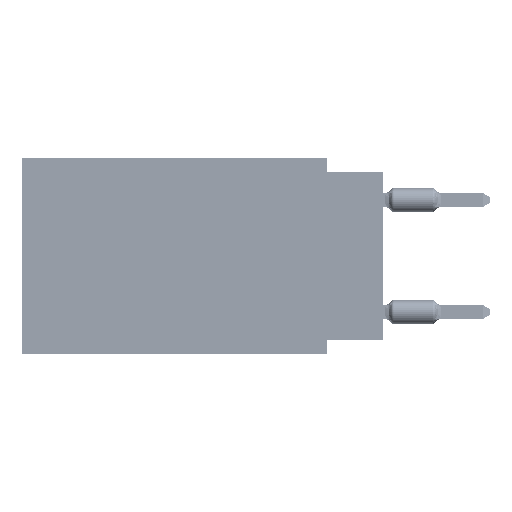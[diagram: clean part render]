
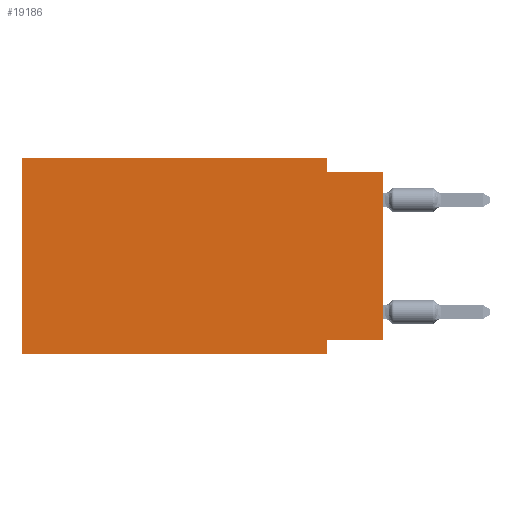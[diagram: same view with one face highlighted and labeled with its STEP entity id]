
A CAD part, left-side view. The second image highlights one B-rep face of the part: STEP entity #19186.
In plain terms, the highlighted planar face has unit normal (-1, 0, 0).
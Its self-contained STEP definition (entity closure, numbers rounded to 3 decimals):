
#31 = EDGE_CURVE ( 'NONE', #23636, #20899, #43520, .T. ) ;
#318 = DIRECTION ( 'NONE',  ( 0., -1., 0. ) ) ;
#2616 = VECTOR ( 'NONE', #43122, 1000. ) ;
#3422 = LINE ( 'NONE', #37999, #2616 ) ;
#3876 = DIRECTION ( 'NONE',  ( 0., 1., 0. ) ) ;
#4145 = VERTEX_POINT ( 'NONE', #33022 ) ;
#4870 = DIRECTION ( 'NONE',  ( 0., -1., 0. ) ) ;
#5807 = CARTESIAN_POINT ( 'NONE',  ( 0., 0., -8.255 ) ) ;
#7226 = EDGE_CURVE ( 'NONE', #23636, #25279, #48385, .T. ) ;
#7866 = ORIENTED_EDGE ( 'NONE', *, *, #9237, .F. ) ;
#8759 = CARTESIAN_POINT ( 'NONE',  ( 0., 2.54, -8.89 ) ) ;
#8992 = DIRECTION ( 'NONE',  ( 0., 0., -1. ) ) ;
#9237 = EDGE_CURVE ( 'NONE', #4145, #21163, #3422, .T. ) ;
#11208 = VECTOR ( 'NONE', #56628, 1000. ) ;
#14123 = CARTESIAN_POINT ( 'NONE',  ( 0., 2.54, -0.635 ) ) ;
#15440 = EDGE_CURVE ( 'NONE', #36112, #4145, #27808, .T. ) ;
#17751 = ORIENTED_EDGE ( 'NONE', *, *, #57872, .F. ) ;
#18705 = PLANE ( 'NONE',  #55763 ) ;
#18850 = LINE ( 'NONE', #56643, #22838 ) ;
#19186 = ADVANCED_FACE ( 'NONE', ( #57759 ), #18705, .F. ) ;
#19490 = DIRECTION ( 'NONE',  ( 0., 0., 1. ) ) ;
#20899 = VERTEX_POINT ( 'NONE', #59959 ) ;
#21163 = VERTEX_POINT ( 'NONE', #14123 ) ;
#22838 = VECTOR ( 'NONE', #62710, 1000. ) ;
#22991 = ORIENTED_EDGE ( 'NONE', *, *, #43922, .F. ) ;
#23264 = VECTOR ( 'NONE', #4870, 1000. ) ;
#23636 = VERTEX_POINT ( 'NONE', #5807 ) ;
#24439 = DIRECTION ( 'NONE',  ( 1., 0., 0. ) ) ;
#24727 = LINE ( 'NONE', #44268, #23264 ) ;
#25279 = VERTEX_POINT ( 'NONE', #49144 ) ;
#26987 = VERTEX_POINT ( 'NONE', #49964 ) ;
#27808 = LINE ( 'NONE', #62074, #11208 ) ;
#32704 = CARTESIAN_POINT ( 'NONE',  ( 0., 2.54, -8.89 ) ) ;
#33021 = EDGE_CURVE ( 'NONE', #26987, #33573, #55367, .T. ) ;
#33022 = CARTESIAN_POINT ( 'NONE',  ( 0., 2.54, 0. ) ) ;
#33269 = CARTESIAN_POINT ( 'NONE',  ( 0., 0., 0. ) ) ;
#33573 = VERTEX_POINT ( 'NONE', #8759 ) ;
#35051 = ORIENTED_EDGE ( 'NONE', *, *, #33021, .T. ) ;
#36112 = VERTEX_POINT ( 'NONE', #41976 ) ;
#37999 = CARTESIAN_POINT ( 'NONE',  ( 0., 2.54, 0. ) ) ;
#38141 = LINE ( 'NONE', #32704, #48024 ) ;
#41038 = EDGE_CURVE ( 'NONE', #21163, #20899, #24727, .T. ) ;
#41687 = ORIENTED_EDGE ( 'NONE', *, *, #31, .T. ) ;
#41976 = CARTESIAN_POINT ( 'NONE',  ( 0., 16.383, 0. ) ) ;
#43122 = DIRECTION ( 'NONE',  ( 0., 0., -1. ) ) ;
#43520 = LINE ( 'NONE', #33269, #57061 ) ;
#43674 = DIRECTION ( 'NONE',  ( 0., 0., -1. ) ) ;
#43922 = EDGE_CURVE ( 'NONE', #26987, #36112, #18850, .T. ) ;
#44180 = VECTOR ( 'NONE', #318, 1000. ) ;
#44268 = CARTESIAN_POINT ( 'NONE',  ( 0., 0., -0.635 ) ) ;
#45804 = ORIENTED_EDGE ( 'NONE', *, *, #7226, .F. ) ;
#48024 = VECTOR ( 'NONE', #8992, 1000. ) ;
#48385 = LINE ( 'NONE', #57352, #51561 ) ;
#48470 = CARTESIAN_POINT ( 'NONE',  ( 0., 16.383, 0. ) ) ;
#49144 = CARTESIAN_POINT ( 'NONE',  ( 0., 2.54, -8.255 ) ) ;
#49964 = CARTESIAN_POINT ( 'NONE',  ( 0., 16.383, -8.89 ) ) ;
#51561 = VECTOR ( 'NONE', #3876, 1000. ) ;
#52772 = EDGE_LOOP ( 'NONE', ( #41687, #54176, #7866, #52896, #22991, #35051, #17751, #45804 ) ) ;
#52896 = ORIENTED_EDGE ( 'NONE', *, *, #15440, .F. ) ;
#54176 = ORIENTED_EDGE ( 'NONE', *, *, #41038, .F. ) ;
#55367 = LINE ( 'NONE', #60186, #44180 ) ;
#55763 = AXIS2_PLACEMENT_3D ( 'NONE', #48470, #24439, #43674 ) ;
#56628 = DIRECTION ( 'NONE',  ( 0., -1., 0. ) ) ;
#56643 = CARTESIAN_POINT ( 'NONE',  ( 0., 16.383, 0. ) ) ;
#57061 = VECTOR ( 'NONE', #19490, 1000. ) ;
#57352 = CARTESIAN_POINT ( 'NONE',  ( 0., 0., -8.255 ) ) ;
#57759 = FACE_OUTER_BOUND ( 'NONE', #52772, .T. ) ;
#57872 = EDGE_CURVE ( 'NONE', #25279, #33573, #38141, .T. ) ;
#59959 = CARTESIAN_POINT ( 'NONE',  ( 0., 0., -0.635 ) ) ;
#60186 = CARTESIAN_POINT ( 'NONE',  ( 0., 16.383, -8.89 ) ) ;
#62074 = CARTESIAN_POINT ( 'NONE',  ( 0., 16.383, 0. ) ) ;
#62710 = DIRECTION ( 'NONE',  ( 0., 0., 1. ) ) ;
